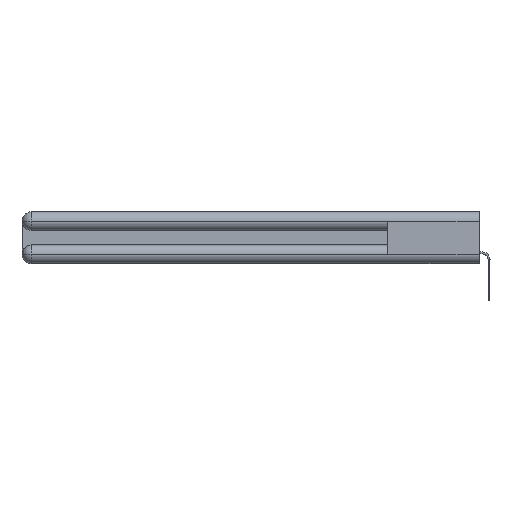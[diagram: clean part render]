
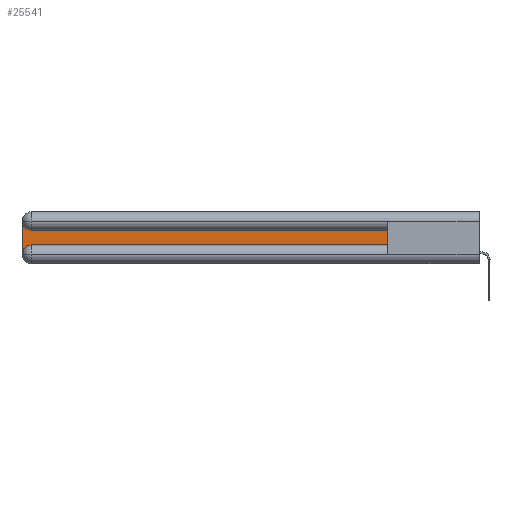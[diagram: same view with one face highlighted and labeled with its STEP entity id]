
A CAD part, left-side view. The second image highlights one B-rep face of the part: STEP entity #25541.
In plain terms, the highlighted planar face has unit normal (-1, 0, 0).
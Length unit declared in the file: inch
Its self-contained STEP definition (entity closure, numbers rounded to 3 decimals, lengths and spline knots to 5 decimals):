
#59 = AXIS2_PLACEMENT_3D ( 'NONE', #11479, #19575, #6986 ) ;
#760 = VERTEX_POINT ( 'NONE', #5045 ) ;
#3884 = CARTESIAN_POINT ( 'NONE',  ( 0.075, 3., -0.1225 ) ) ;
#4288 = VECTOR ( 'NONE', #24819, 39.37008 ) ;
#4318 = VERTEX_POINT ( 'NONE', #15782 ) ;
#5045 = CARTESIAN_POINT ( 'NONE',  ( 0.075, 2.94, -0.1225 ) ) ;
#5056 = ORIENTED_EDGE ( 'NONE', *, *, #16792, .T. ) ;
#6154 = VERTEX_POINT ( 'NONE', #23605 ) ;
#6986 = DIRECTION ( 'NONE',  ( 0., 0., -1. ) ) ;
#8290 = EDGE_CURVE ( 'NONE', #21501, #19876, #23913, .T. ) ;
#8551 = ORIENTED_EDGE ( 'NONE', *, *, #26057, .T. ) ;
#10142 = ORIENTED_EDGE ( 'NONE', *, *, #18311, .T. ) ;
#10191 = LINE ( 'NONE', #18549, #4288 ) ;
#10764 = CARTESIAN_POINT ( 'NONE',  ( 0.075, 2.94, -0.2175 ) ) ;
#10962 = CIRCLE ( 'NONE', #59, 0.06 ) ;
#11077 = ORIENTED_EDGE ( 'NONE', *, *, #16927, .T. ) ;
#11150 = CARTESIAN_POINT ( 'NONE',  ( 0.075, 3., -0.2775 ) ) ;
#11235 = DIRECTION ( 'NONE',  ( 0., 0., -1. ) ) ;
#11479 = CARTESIAN_POINT ( 'NONE',  ( 0.075, 2.94, -0.0625 ) ) ;
#11944 = PLANE ( 'NONE',  #17712 ) ;
#12982 = ORIENTED_EDGE ( 'NONE', *, *, #15055, .T. ) ;
#13440 = AXIS2_PLACEMENT_3D ( 'NONE', #23679, #21371, #11235 ) ;
#13713 = VECTOR ( 'NONE', #20333, 39.37008 ) ;
#13743 = FACE_OUTER_BOUND ( 'NONE', #25420, .T. ) ;
#15045 = VERTEX_POINT ( 'NONE', #27009 ) ;
#15055 = EDGE_CURVE ( 'NONE', #4318, #21501, #10191, .T. ) ;
#15782 = CARTESIAN_POINT ( 'NONE',  ( 0.075, 3., -0.0625 ) ) ;
#16792 = EDGE_CURVE ( 'NONE', #15045, #760, #18606, .T. ) ;
#16868 = VECTOR ( 'NONE', #23208, 39.37008 ) ;
#16927 = EDGE_CURVE ( 'NONE', #19876, #6154, #23921, .T. ) ;
#16943 = LINE ( 'NONE', #23344, #16868 ) ;
#17712 = AXIS2_PLACEMENT_3D ( 'NONE', #3884, #20553, #20299 ) ;
#18311 = EDGE_CURVE ( 'NONE', #760, #4318, #10962, .T. ) ;
#18549 = CARTESIAN_POINT ( 'NONE',  ( 0.075, 3., -0.2175 ) ) ;
#18606 = LINE ( 'NONE', #20385, #22431 ) ;
#19575 = DIRECTION ( 'NONE',  ( 1., 0., 0. ) ) ;
#19876 = VERTEX_POINT ( 'NONE', #10764 ) ;
#20299 = DIRECTION ( 'NONE',  ( 0., 0., -1. ) ) ;
#20333 = DIRECTION ( 'NONE',  ( 0., -1., 0. ) ) ;
#20385 = CARTESIAN_POINT ( 'NONE',  ( 0.075, 0.6, -0.1225 ) ) ;
#20516 = DIRECTION ( 'NONE',  ( 0., 1., 0. ) ) ;
#20553 = DIRECTION ( 'NONE',  ( 1., 0., 0. ) ) ;
#21371 = DIRECTION ( 'NONE',  ( 1., 0., 0. ) ) ;
#21501 = VERTEX_POINT ( 'NONE', #11150 ) ;
#21565 = ORIENTED_EDGE ( 'NONE', *, *, #8290, .T. ) ;
#22431 = VECTOR ( 'NONE', #20516, 39.37008 ) ;
#23208 = DIRECTION ( 'NONE',  ( 0., 0., 1. ) ) ;
#23344 = CARTESIAN_POINT ( 'NONE',  ( 0.075, 0.6, -0.2175 ) ) ;
#23605 = CARTESIAN_POINT ( 'NONE',  ( 0.075, 0.6, -0.2175 ) ) ;
#23679 = CARTESIAN_POINT ( 'NONE',  ( 0.075, 2.94, -0.2775 ) ) ;
#23913 = CIRCLE ( 'NONE', #13440, 0.06 ) ;
#23921 = LINE ( 'NONE', #25824, #13713 ) ;
#24819 = DIRECTION ( 'NONE',  ( 0., 0., -1. ) ) ;
#25420 = EDGE_LOOP ( 'NONE', ( #5056, #10142, #12982, #21565, #11077, #8551 ) ) ;
#25541 = ADVANCED_FACE ( 'NONE', ( #13743 ), #11944, .F. ) ;
#25824 = CARTESIAN_POINT ( 'NONE',  ( 0.075, 0.6, -0.2175 ) ) ;
#26057 = EDGE_CURVE ( 'NONE', #6154, #15045, #16943, .T. ) ;
#27009 = CARTESIAN_POINT ( 'NONE',  ( 0.075, 0.6, -0.1225 ) ) ;
